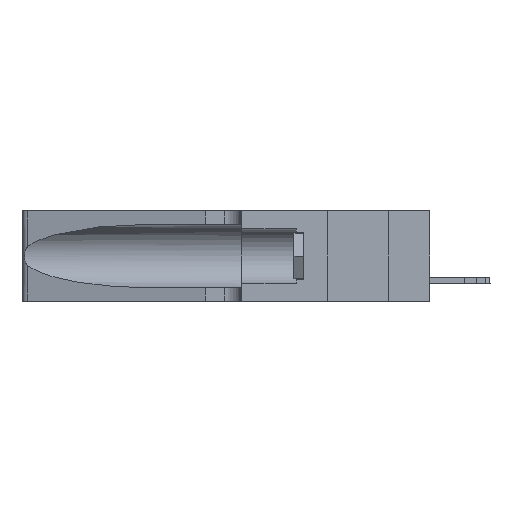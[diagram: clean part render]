
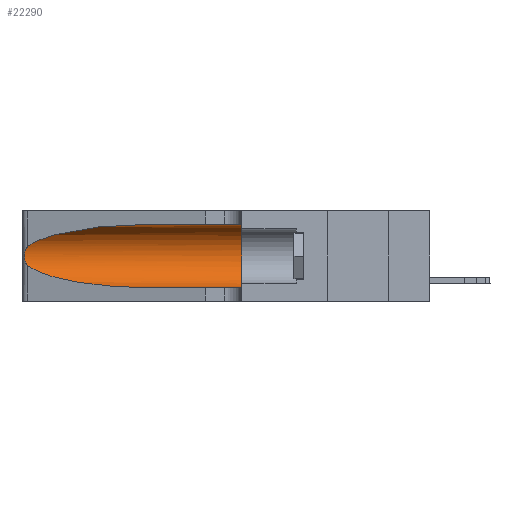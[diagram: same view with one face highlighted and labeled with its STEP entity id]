
A CAD part, left-side view. The second image highlights one B-rep face of the part: STEP entity #22290.
In plain terms, the highlighted cylindrical face has radius 3.308 mm (diameter 6.617 mm), a partial arc.
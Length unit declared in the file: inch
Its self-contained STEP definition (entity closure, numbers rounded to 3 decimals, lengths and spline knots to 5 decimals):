
#557 = CIRCLE ( 'NONE', #19479, 0.13025 ) ;
#1080 = CARTESIAN_POINT ( 'NONE',  ( 0.1305, 0.72297, 0.05475 ) ) ;
#1696 = CARTESIAN_POINT ( 'NONE',  ( 0.25789, 1.23486, 0.15765 ) ) ;
#1705 = VERTEX_POINT ( 'NONE', #6998 ) ;
#1786 = CARTESIAN_POINT ( 'NONE',  ( 0.25555, 1.22994, 0.2215 ) ) ;
#2221 = DIRECTION ( 'NONE',  ( 0., -1., 0. ) ) ;
#2322 = ORIENTED_EDGE ( 'NONE', *, *, #15028, .T. ) ;
#2392 = CARTESIAN_POINT ( 'NONE',  ( 0.1305, 1.61858, 0.31525 ) ) ;
#3515 = CARTESIAN_POINT ( 'NONE',  ( 0.26075, 1.23896, 0.19203 ) ) ;
#3536 = ORIENTED_EDGE ( 'NONE', *, *, #25576, .F. ) ;
#3580 = DIRECTION ( 'NONE',  ( 0., 1., 0. ) ) ;
#4540 = CARTESIAN_POINT ( 'NONE',  ( 0.1305, 1.61858, 0.05475 ) ) ;
#4685 = CARTESIAN_POINT ( 'NONE',  ( 0.1305, 0.35, 0.31525 ) ) ;
#5404 = ORIENTED_EDGE ( 'NONE', *, *, #24017, .T. ) ;
#5560 = EDGE_LOOP ( 'NONE', ( #2322, #6244, #5404, #20449, #19493, #3536 ) ) ;
#5573 = DIRECTION ( 'NONE',  ( 0., 0., 1. ) ) ;
#6244 = ORIENTED_EDGE ( 'NONE', *, *, #24195, .T. ) ;
#6998 = CARTESIAN_POINT ( 'NONE',  ( 0.25487, 1.22718, 0.22369 ) ) ;
#7550 = AXIS2_PLACEMENT_3D ( 'NONE', #23458, #25452, #23544 ) ;
#7609 = CARTESIAN_POINT ( 'NONE',  ( 0.25487, 1.22718, 0.22369 ) ) ;
#7708 = CARTESIAN_POINT ( 'NONE',  ( 0.25555, 1.22993, 0.14849 ) ) ;
#8197 = CYLINDRICAL_SURFACE ( 'NONE', #7550, 0.13025 ) ;
#8631 = VERTEX_POINT ( 'NONE', #13879 ) ;
#8783 = CARTESIAN_POINT ( 'NONE',  ( 0.25487, 1.22718, 0.14631 ) ) ;
#9332 = CARTESIAN_POINT ( 'NONE',  ( 0.18966, 0.96281, 0.05475 ) ) ;
#9621 = CARTESIAN_POINT ( 'NONE',  ( 0.1305, 0.72297, 0.05475 ) ) ;
#9767 = CARTESIAN_POINT ( 'NONE',  ( 0.25487, 1.22718, 0.14631 ) ) ;
#9919 = VECTOR ( 'NONE', #10552, 39.37008 ) ;
#10552 = DIRECTION ( 'NONE',  ( 0., -1., 0. ) ) ;
#10849 = LINE ( 'NONE', #4540, #9919 ) ;
#11331 = CARTESIAN_POINT ( 'NONE',  ( 0.2373, 1.15595, 0.28018 ) ) ;
#11701 = CARTESIAN_POINT ( 'NONE',  ( 0.25856, 1.23593, 0.16098 ) ) ;
#12454 =( BOUNDED_CURVE ( )  B_SPLINE_CURVE ( 3, ( #24779, #12801, #9332, #1080 ),
 .UNSPECIFIED., .F., .T. ) 
 B_SPLINE_CURVE_WITH_KNOTS ( ( 4, 4 ),
 ( 3.44316, 4.71239 ),
 .UNSPECIFIED. ) 
 CURVE ( )  GEOMETRIC_REPRESENTATION_ITEM ( )  RATIONAL_B_SPLINE_CURVE ( ( 1., 0.87, 0.87, 1. ) ) 
 REPRESENTATION_ITEM ( '' )  );
#12504 = CARTESIAN_POINT ( 'NONE',  ( 0.1305, 0.72297, 0.31525 ) ) ;
#12688 = VECTOR ( 'NONE', #2221, 39.37008 ) ;
#12801 = CARTESIAN_POINT ( 'NONE',  ( 0.2373, 1.15595, 0.08982 ) ) ;
#13607 = CARTESIAN_POINT ( 'NONE',  ( 0.26075, 1.23896, 0.178 ) ) ;
#13879 = CARTESIAN_POINT ( 'NONE',  ( 0.1305, 0.35, 0.05475 ) ) ;
#15028 = EDGE_CURVE ( 'NONE', #20622, #1705, #21781, .T. ) ;
#15165 = CARTESIAN_POINT ( 'NONE',  ( 0.1305, 0.72297, 0.31525 ) ) ;
#15476 = CARTESIAN_POINT ( 'NONE',  ( 0.1305, 0.35, 0.185 ) ) ;
#16921 = FACE_OUTER_BOUND ( 'NONE', #5560, .T. ) ;
#19479 = AXIS2_PLACEMENT_3D ( 'NONE', #15476, #3580, #5573 ) ;
#19493 = ORIENTED_EDGE ( 'NONE', *, *, #24930, .F. ) ;
#19650 = CARTESIAN_POINT ( 'NONE',  ( 0.25639, 1.23186, 0.15144 ) ) ;
#20035 = VERTEX_POINT ( 'NONE', #8783 ) ;
#20449 = ORIENTED_EDGE ( 'NONE', *, *, #21554, .T. ) ;
#20575 = VERTEX_POINT ( 'NONE', #4685 ) ;
#20622 = VERTEX_POINT ( 'NONE', #12504 ) ;
#20971 = B_SPLINE_CURVE_WITH_KNOTS ( 'NONE', 3,
 ( #7609, #1786, #21561, #25718, #25549, #23571, #3515, #13607, #25633, #11701, #1696, #19650, #7708, #9767 ),
 .UNSPECIFIED., .F., .F.,
 ( 4, 2, 2, 2, 2, 2, 4 ),
 ( 0., 0.00027, 0.00053, 0.00107, 0.0016, 0.00187, 0.00214 ),
 .UNSPECIFIED. ) ;
#21378 = CARTESIAN_POINT ( 'NONE',  ( 0.18966, 0.96281, 0.31525 ) ) ;
#21554 = EDGE_CURVE ( 'NONE', #23648, #8631, #10849, .T. ) ;
#21561 = CARTESIAN_POINT ( 'NONE',  ( 0.25639, 1.23184, 0.21858 ) ) ;
#21781 =( BOUNDED_CURVE ( )  B_SPLINE_CURVE ( 3, ( #15165, #21378, #11331, #23566 ),
 .UNSPECIFIED., .F., .T. ) 
 B_SPLINE_CURVE_WITH_KNOTS ( ( 4, 4 ),
 ( 1.5708, 2.84003 ),
 .UNSPECIFIED. ) 
 CURVE ( )  GEOMETRIC_REPRESENTATION_ITEM ( )  RATIONAL_B_SPLINE_CURVE ( ( 1., 0.87, 0.87, 1. ) ) 
 REPRESENTATION_ITEM ( '' )  );
#22290 = ADVANCED_FACE ( 'NONE', ( #16921 ), #8197, .F. ) ;
#22405 = LINE ( 'NONE', #2392, #12688 ) ;
#23458 = CARTESIAN_POINT ( 'NONE',  ( 0.1305, 1.61858, 0.185 ) ) ;
#23544 = DIRECTION ( 'NONE',  ( 0., 0., -1. ) ) ;
#23566 = CARTESIAN_POINT ( 'NONE',  ( 0.25487, 1.22718, 0.22369 ) ) ;
#23571 = CARTESIAN_POINT ( 'NONE',  ( 0.26018, 1.23835, 0.19895 ) ) ;
#23648 = VERTEX_POINT ( 'NONE', #9621 ) ;
#24017 = EDGE_CURVE ( 'NONE', #20035, #23648, #12454, .T. ) ;
#24195 = EDGE_CURVE ( 'NONE', #1705, #20035, #20971, .T. ) ;
#24779 = CARTESIAN_POINT ( 'NONE',  ( 0.25487, 1.22718, 0.14631 ) ) ;
#24930 = EDGE_CURVE ( 'NONE', #20575, #8631, #557, .T. ) ;
#25452 = DIRECTION ( 'NONE',  ( 0., -1., 0. ) ) ;
#25549 = CARTESIAN_POINT ( 'NONE',  ( 0.25854, 1.2359, 0.20912 ) ) ;
#25576 = EDGE_CURVE ( 'NONE', #20622, #20575, #22405, .T. ) ;
#25633 = CARTESIAN_POINT ( 'NONE',  ( 0.26017, 1.23833, 0.17102 ) ) ;
#25718 = CARTESIAN_POINT ( 'NONE',  ( 0.25787, 1.23484, 0.2124 ) ) ;
